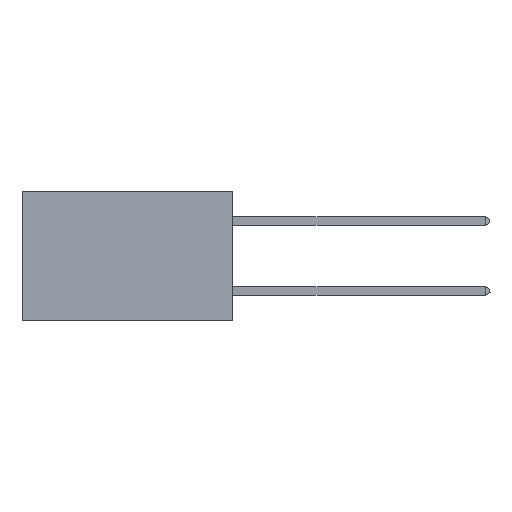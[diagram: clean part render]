
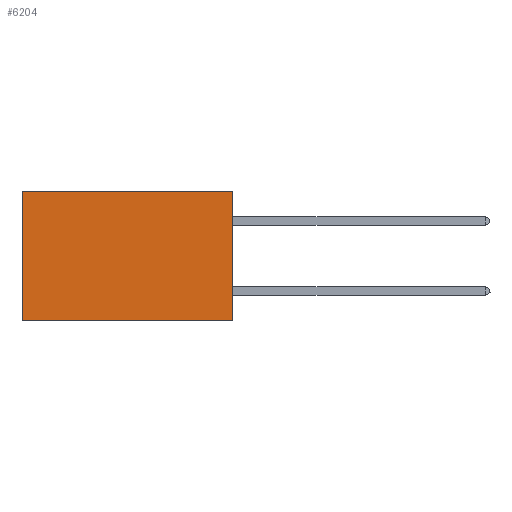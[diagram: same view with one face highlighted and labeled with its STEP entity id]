
A CAD part, left-side view. The second image highlights one B-rep face of the part: STEP entity #6204.
In plain terms, the highlighted planar face has unit normal (-1, 0, 0).
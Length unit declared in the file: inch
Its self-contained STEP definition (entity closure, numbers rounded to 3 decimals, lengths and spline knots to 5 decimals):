
#48 = EDGE_CURVE ( 'NONE', #7604, #16411, #4129, .T. ) ;
#118 = CARTESIAN_POINT ( 'NONE',  ( 0.2875, 0., 0. ) ) ;
#1271 = CARTESIAN_POINT ( 'NONE',  ( 0.2875, 0., 0. ) ) ;
#1565 = VECTOR ( 'NONE', #8893, 39.37008 ) ;
#1671 = CARTESIAN_POINT ( 'NONE',  ( 0.2875, 0.6, -0.37 ) ) ;
#1774 = CARTESIAN_POINT ( 'NONE',  ( 0.2875, 0., 0. ) ) ;
#2674 = PLANE ( 'NONE',  #11298 ) ;
#2697 = EDGE_LOOP ( 'NONE', ( #4333, #14339, #17745, #14733 ) ) ;
#3238 = VECTOR ( 'NONE', #10391, 39.37008 ) ;
#3909 = VECTOR ( 'NONE', #9690, 39.37008 ) ;
#4129 = LINE ( 'NONE', #8239, #3909 ) ;
#4321 = FACE_OUTER_BOUND ( 'NONE', #2697, .T. ) ;
#4333 = ORIENTED_EDGE ( 'NONE', *, *, #5740, .T. ) ;
#5740 = EDGE_CURVE ( 'NONE', #8348, #16411, #6441, .T. ) ;
#6192 = EDGE_CURVE ( 'NONE', #11823, #8348, #10759, .T. ) ;
#6204 = ADVANCED_FACE ( 'NONE', ( #4321 ), #2674, .F. ) ;
#6441 = LINE ( 'NONE', #10236, #13544 ) ;
#7378 = CARTESIAN_POINT ( 'NONE',  ( 0.2875, 0., 0. ) ) ;
#7604 = VERTEX_POINT ( 'NONE', #18107 ) ;
#8239 = CARTESIAN_POINT ( 'NONE',  ( 0.2875, 0., -0.37 ) ) ;
#8348 = VERTEX_POINT ( 'NONE', #15461 ) ;
#8893 = DIRECTION ( 'NONE',  ( 0., 1., 0. ) ) ;
#9690 = DIRECTION ( 'NONE',  ( 0., 1., 0. ) ) ;
#10236 = CARTESIAN_POINT ( 'NONE',  ( 0.2875, 0.6, 0. ) ) ;
#10391 = DIRECTION ( 'NONE',  ( 0., 0., -1. ) ) ;
#10759 = LINE ( 'NONE', #1774, #1565 ) ;
#11298 = AXIS2_PLACEMENT_3D ( 'NONE', #1271, #11636, #18891 ) ;
#11636 = DIRECTION ( 'NONE',  ( 1., 0., 0. ) ) ;
#11823 = VERTEX_POINT ( 'NONE', #7378 ) ;
#13448 = DIRECTION ( 'NONE',  ( 0., 0., -1. ) ) ;
#13544 = VECTOR ( 'NONE', #13448, 39.37008 ) ;
#14339 = ORIENTED_EDGE ( 'NONE', *, *, #48, .F. ) ;
#14733 = ORIENTED_EDGE ( 'NONE', *, *, #6192, .T. ) ;
#15461 = CARTESIAN_POINT ( 'NONE',  ( 0.2875, 0.6, 0. ) ) ;
#16411 = VERTEX_POINT ( 'NONE', #1671 ) ;
#17292 = LINE ( 'NONE', #118, #3238 ) ;
#17550 = EDGE_CURVE ( 'NONE', #11823, #7604, #17292, .T. ) ;
#17745 = ORIENTED_EDGE ( 'NONE', *, *, #17550, .F. ) ;
#18107 = CARTESIAN_POINT ( 'NONE',  ( 0.2875, 0., -0.37 ) ) ;
#18891 = DIRECTION ( 'NONE',  ( 0., 0., -1. ) ) ;
